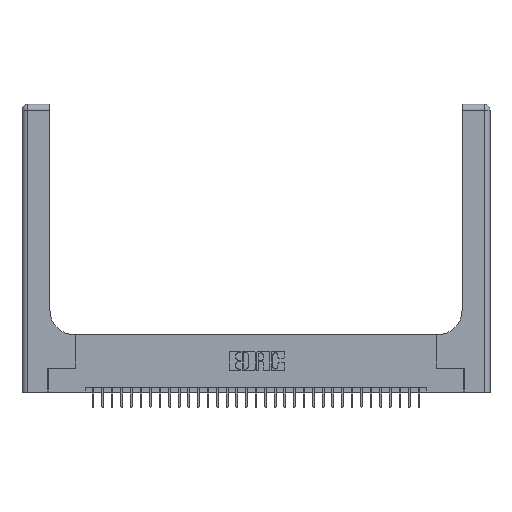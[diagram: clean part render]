
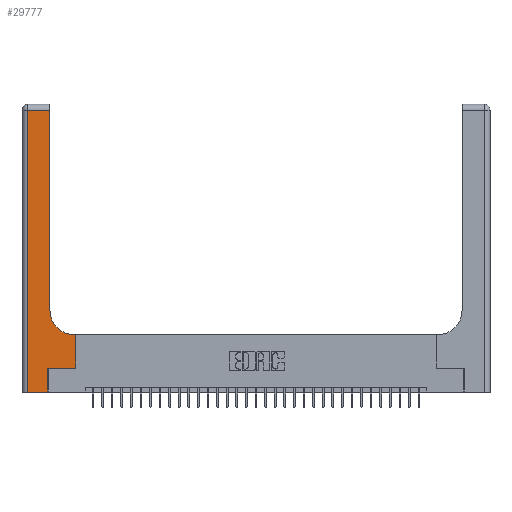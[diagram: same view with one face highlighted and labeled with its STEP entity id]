
A CAD part, top view. The second image highlights one B-rep face of the part: STEP entity #29777.
In plain terms, the highlighted planar face has unit normal (0, 0, 1).
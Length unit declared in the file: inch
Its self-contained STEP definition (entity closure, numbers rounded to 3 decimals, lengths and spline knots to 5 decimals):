
#195 = CARTESIAN_POINT ( 'NONE',  ( 0.5585, 0.25, 0.37 ) ) ;
#399 = VECTOR ( 'NONE', #8573, 39.37008 ) ;
#678 = DIRECTION ( 'NONE',  ( 0., -1., 0. ) ) ;
#1540 = ORIENTED_EDGE ( 'NONE', *, *, #28117, .T. ) ;
#2078 = LINE ( 'NONE', #18952, #399 ) ;
#2241 = VECTOR ( 'NONE', #20764, 39.37008 ) ;
#2608 = EDGE_CURVE ( 'NONE', #33033, #7612, #2078, .T. ) ;
#2684 = CARTESIAN_POINT ( 'NONE',  ( 0., 0., 0.37 ) ) ;
#3006 = ORIENTED_EDGE ( 'NONE', *, *, #25198, .T. ) ;
#3278 = ORIENTED_EDGE ( 'NONE', *, *, #20292, .T. ) ;
#4069 = VERTEX_POINT ( 'NONE', #16925 ) ;
#4362 = VERTEX_POINT ( 'NONE', #23318 ) ;
#4531 = AXIS2_PLACEMENT_3D ( 'NONE', #5419, #23598, #8092 ) ;
#4783 = VECTOR ( 'NONE', #23227, 39.37008 ) ;
#5030 = CIRCLE ( 'NONE', #4531, 0.25 ) ;
#5409 = CARTESIAN_POINT ( 'NONE',  ( 0.5585, 0.6, 0.37 ) ) ;
#5419 = CARTESIAN_POINT ( 'NONE',  ( 0.5415, 0.85, 0.37 ) ) ;
#6465 = DIRECTION ( 'NONE',  ( 1., 0., 0. ) ) ;
#6627 = DIRECTION ( 'NONE',  ( 0., 1., 0. ) ) ;
#7612 = VERTEX_POINT ( 'NONE', #5409 ) ;
#8092 = DIRECTION ( 'NONE',  ( 1., 0., 0. ) ) ;
#8247 = VERTEX_POINT ( 'NONE', #14211 ) ;
#8573 = DIRECTION ( 'NONE',  ( 0., 1., 0. ) ) ;
#9338 = VERTEX_POINT ( 'NONE', #18549 ) ;
#9381 = ORIENTED_EDGE ( 'NONE', *, *, #32972, .T. ) ;
#9977 = ORIENTED_EDGE ( 'NONE', *, *, #2608, .T. ) ;
#10223 = LINE ( 'NONE', #28317, #2241 ) ;
#10536 = FACE_OUTER_BOUND ( 'NONE', #14431, .T. ) ;
#10715 = EDGE_CURVE ( 'NONE', #21965, #27199, #24629, .T. ) ;
#11007 = LINE ( 'NONE', #25675, #4783 ) ;
#11248 = CARTESIAN_POINT ( 'NONE',  ( 0.06, 2.94, 0.37 ) ) ;
#11331 = CARTESIAN_POINT ( 'NONE',  ( 0.06, 3., 0.37 ) ) ;
#14211 = CARTESIAN_POINT ( 'NONE',  ( 0.269, 0.25, 0.37 ) ) ;
#14431 = EDGE_LOOP ( 'NONE', ( #1540, #28090, #32019, #9381, #3278, #26428, #9977, #15915, #3006 ) ) ;
#14774 = CARTESIAN_POINT ( 'NONE',  ( 0.2915, 0.6, 0.37 ) ) ;
#15228 = EDGE_CURVE ( 'NONE', #4362, #21965, #11007, .T. ) ;
#15397 = AXIS2_PLACEMENT_3D ( 'NONE', #31385, #31489, #16146 ) ;
#15679 = EDGE_CURVE ( 'NONE', #7612, #9338, #30667, .T. ) ;
#15915 = ORIENTED_EDGE ( 'NONE', *, *, #15679, .T. ) ;
#16146 = DIRECTION ( 'NONE',  ( -1., 0., 0. ) ) ;
#16864 = CARTESIAN_POINT ( 'NONE',  ( 0.269, 0.25, 0.37 ) ) ;
#16891 = CARTESIAN_POINT ( 'NONE',  ( 0.269, 0., 0.37 ) ) ;
#16925 = CARTESIAN_POINT ( 'NONE',  ( 0.2915, 0.85, 0.37 ) ) ;
#17806 = VECTOR ( 'NONE', #678, 39.37008 ) ;
#18549 = CARTESIAN_POINT ( 'NONE',  ( 0.5415, 0.6, 0.37 ) ) ;
#18578 = LINE ( 'NONE', #16864, #23771 ) ;
#18952 = CARTESIAN_POINT ( 'NONE',  ( 0.5585, 0.25, 0.37 ) ) ;
#19653 = CARTESIAN_POINT ( 'NONE',  ( 0.269, 0., 0.37 ) ) ;
#20255 = LINE ( 'NONE', #19653, #32179 ) ;
#20292 = EDGE_CURVE ( 'NONE', #28602, #8247, #20255, .T. ) ;
#20764 = DIRECTION ( 'NONE',  ( 0., 1., 0. ) ) ;
#20870 = EDGE_CURVE ( 'NONE', #8247, #33033, #18578, .T. ) ;
#21965 = VERTEX_POINT ( 'NONE', #11248 ) ;
#23227 = DIRECTION ( 'NONE',  ( -1., 0., 0. ) ) ;
#23318 = CARTESIAN_POINT ( 'NONE',  ( 0.2915, 2.94, 0.37 ) ) ;
#23598 = DIRECTION ( 'NONE',  ( 0., 0., -1. ) ) ;
#23604 = DIRECTION ( 'NONE',  ( 1., 0., 0. ) ) ;
#23771 = VECTOR ( 'NONE', #6465, 39.37008 ) ;
#24533 = VECTOR ( 'NONE', #23604, 39.37008 ) ;
#24629 = LINE ( 'NONE', #11331, #17806 ) ;
#25198 = EDGE_CURVE ( 'NONE', #9338, #4069, #5030, .T. ) ;
#25675 = CARTESIAN_POINT ( 'NONE',  ( 0., 2.94, 0.37 ) ) ;
#26354 = PLANE ( 'NONE',  #15397 ) ;
#26428 = ORIENTED_EDGE ( 'NONE', *, *, #20870, .T. ) ;
#27199 = VERTEX_POINT ( 'NONE', #29262 ) ;
#28090 = ORIENTED_EDGE ( 'NONE', *, *, #15228, .T. ) ;
#28117 = EDGE_CURVE ( 'NONE', #4069, #4362, #10223, .T. ) ;
#28317 = CARTESIAN_POINT ( 'NONE',  ( 0.2915, 3., 0.37 ) ) ;
#28602 = VERTEX_POINT ( 'NONE', #16891 ) ;
#29262 = CARTESIAN_POINT ( 'NONE',  ( 0.06, 0., 0.37 ) ) ;
#29777 = ADVANCED_FACE ( 'NONE', ( #10536 ), #26354, .F. ) ;
#29872 = VECTOR ( 'NONE', #30132, 39.37008 ) ;
#30132 = DIRECTION ( 'NONE',  ( -1., 0., 0. ) ) ;
#30667 = LINE ( 'NONE', #14774, #29872 ) ;
#31313 = LINE ( 'NONE', #2684, #24533 ) ;
#31385 = CARTESIAN_POINT ( 'NONE',  ( 0., 3., 0.37 ) ) ;
#31489 = DIRECTION ( 'NONE',  ( 0., 0., -1. ) ) ;
#32019 = ORIENTED_EDGE ( 'NONE', *, *, #10715, .T. ) ;
#32179 = VECTOR ( 'NONE', #6627, 39.37008 ) ;
#32972 = EDGE_CURVE ( 'NONE', #27199, #28602, #31313, .T. ) ;
#33033 = VERTEX_POINT ( 'NONE', #195 ) ;
